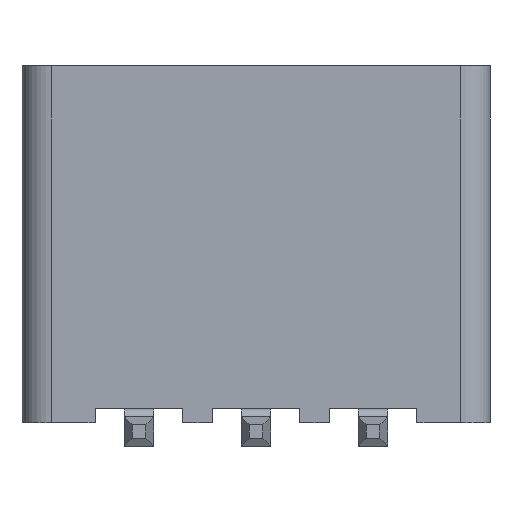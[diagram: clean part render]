
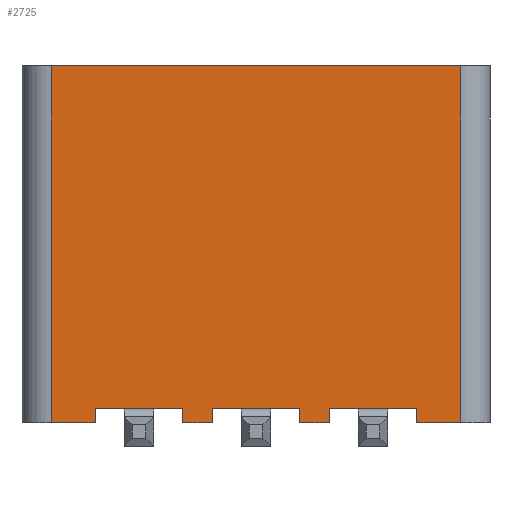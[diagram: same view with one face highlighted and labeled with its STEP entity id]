
A CAD part, front view. The second image highlights one B-rep face of the part: STEP entity #2725.
In plain terms, the highlighted planar face has unit normal (0, -1, 0).
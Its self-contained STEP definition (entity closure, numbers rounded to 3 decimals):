
#11 = ORIENTED_EDGE ( 'NONE', *, *, #2020, .T. ) ;
#19 = CARTESIAN_POINT ( 'NONE',  ( 4.75, -2.7, 0. ) ) ;
#38 = VECTOR ( 'NONE', #557, 1000. ) ;
#58 = LINE ( 'NONE', #2174, #2047 ) ;
#85 = LINE ( 'NONE', #789, #38 ) ;
#87 = LINE ( 'NONE', #790, #674 ) ;
#128 = CARTESIAN_POINT ( 'NONE',  ( 1.25, -2.7, 0.25 ) ) ;
#173 = EDGE_CURVE ( 'NONE', #2019, #825, #58, .T. ) ;
#180 = EDGE_CURVE ( 'NONE', #424, #192, #2599, .T. ) ;
#192 = VERTEX_POINT ( 'NONE', #19 ) ;
#199 = CARTESIAN_POINT ( 'NONE',  ( 5.5, -2.7, 6.1 ) ) ;
#227 = DIRECTION ( 'NONE',  ( 0., 0., -1. ) ) ;
#266 = ORIENTED_EDGE ( 'NONE', *, *, #180, .T. ) ;
#269 = EDGE_CURVE ( 'NONE', #2885, #192, #536, .T. ) ;
#272 = CARTESIAN_POINT ( 'NONE',  ( 3.25, -2.7, 0.25 ) ) ;
#284 = CARTESIAN_POINT ( 'NONE',  ( 2.75, -2.7, 0. ) ) ;
#292 = ORIENTED_EDGE ( 'NONE', *, *, #2459, .F. ) ;
#300 = EDGE_CURVE ( 'NONE', #2869, #2008, #2624, .T. ) ;
#386 = CARTESIAN_POINT ( 'NONE',  ( -0.75, -2.7, 0. ) ) ;
#424 = VERTEX_POINT ( 'NONE', #2438 ) ;
#430 = VECTOR ( 'NONE', #1028, 1000. ) ;
#444 = LINE ( 'NONE', #199, #855 ) ;
#485 = EDGE_CURVE ( 'NONE', #1780, #424, #2649, .T. ) ;
#536 = LINE ( 'NONE', #1696, #2934 ) ;
#546 = VECTOR ( 'NONE', #2665, 1000. ) ;
#548 = ORIENTED_EDGE ( 'NONE', *, *, #2623, .T. ) ;
#557 = DIRECTION ( 'NONE',  ( -1., 0., 0. ) ) ;
#564 = VECTOR ( 'NONE', #2531, 1000. ) ;
#566 = VECTOR ( 'NONE', #834, 1000. ) ;
#576 = DIRECTION ( 'NONE',  ( 0., 0., -1. ) ) ;
#588 = VERTEX_POINT ( 'NONE', #1797 ) ;
#674 = VECTOR ( 'NONE', #2382, 1000. ) ;
#732 = DIRECTION ( 'NONE',  ( 0., 0., 1. ) ) ;
#789 = CARTESIAN_POINT ( 'NONE',  ( 6., -2.7, 0. ) ) ;
#790 = CARTESIAN_POINT ( 'NONE',  ( 6., -2.7, 0. ) ) ;
#803 = LINE ( 'NONE', #2239, #2181 ) ;
#825 = VERTEX_POINT ( 'NONE', #2109 ) ;
#827 = EDGE_CURVE ( 'NONE', #2881, #2975, #3008, .T. ) ;
#834 = DIRECTION ( 'NONE',  ( 1., 0., 0. ) ) ;
#855 = VECTOR ( 'NONE', #1823, 1000. ) ;
#888 = CARTESIAN_POINT ( 'NONE',  ( 2.75, -2.7, 0.25 ) ) ;
#971 = EDGE_CURVE ( 'NONE', #2869, #2089, #85, .T. ) ;
#1028 = DIRECTION ( 'NONE',  ( 0., 0., 1. ) ) ;
#1059 = DIRECTION ( 'NONE',  ( 0., -1., 0. ) ) ;
#1067 = EDGE_CURVE ( 'NONE', #2348, #1780, #2000, .T. ) ;
#1071 = CARTESIAN_POINT ( 'NONE',  ( 2.75, -2.7, 0.25 ) ) ;
#1079 = VERTEX_POINT ( 'NONE', #1982 ) ;
#1122 = EDGE_CURVE ( 'NONE', #2106, #825, #1556, .T. ) ;
#1140 = CARTESIAN_POINT ( 'NONE',  ( -0.75, -2.7, 0.25 ) ) ;
#1199 = VECTOR ( 'NONE', #732, 1000. ) ;
#1203 = VECTOR ( 'NONE', #1545, 1000. ) ;
#1235 = CARTESIAN_POINT ( 'NONE',  ( 1.25, -2.7, 0.25 ) ) ;
#1263 = CARTESIAN_POINT ( 'NONE',  ( 3.25, -2.7, 0. ) ) ;
#1285 = CARTESIAN_POINT ( 'NONE',  ( 6., -2.7, 6.1 ) ) ;
#1304 = EDGE_CURVE ( 'NONE', #1642, #588, #2763, .T. ) ;
#1313 = DIRECTION ( 'NONE',  ( 0., 0., 1. ) ) ;
#1360 = AXIS2_PLACEMENT_3D ( 'NONE', #1285, #1059, #1375 ) ;
#1375 = DIRECTION ( 'NONE',  ( 0., 0., 1. ) ) ;
#1511 = FACE_OUTER_BOUND ( 'NONE', #2034, .T. ) ;
#1515 = EDGE_CURVE ( 'NONE', #1079, #2106, #2484, .T. ) ;
#1516 = CARTESIAN_POINT ( 'NONE',  ( 6., -2.7, 6.1 ) ) ;
#1526 = CARTESIAN_POINT ( 'NONE',  ( -0.75, -2.7, 0.25 ) ) ;
#1545 = DIRECTION ( 'NONE',  ( 0., 0., -1. ) ) ;
#1556 = LINE ( 'NONE', #2014, #1203 ) ;
#1580 = EDGE_CURVE ( 'NONE', #588, #2089, #803, .T. ) ;
#1608 = EDGE_CURVE ( 'NONE', #2885, #1079, #444, .T. ) ;
#1621 = ORIENTED_EDGE ( 'NONE', *, *, #827, .T. ) ;
#1642 = VERTEX_POINT ( 'NONE', #1140 ) ;
#1690 = CARTESIAN_POINT ( 'NONE',  ( 4.75, -2.7, 0.25 ) ) ;
#1696 = CARTESIAN_POINT ( 'NONE',  ( 6., -2.7, 0. ) ) ;
#1733 = LINE ( 'NONE', #1526, #2654 ) ;
#1752 = VECTOR ( 'NONE', #227, 1000. ) ;
#1780 = VERTEX_POINT ( 'NONE', #272 ) ;
#1797 = CARTESIAN_POINT ( 'NONE',  ( 0.75, -2.7, 0.25 ) ) ;
#1823 = DIRECTION ( 'NONE',  ( 0., 0., 1. ) ) ;
#1835 = ORIENTED_EDGE ( 'NONE', *, *, #1608, .T. ) ;
#1900 = ORIENTED_EDGE ( 'NONE', *, *, #485, .T. ) ;
#1926 = CARTESIAN_POINT ( 'NONE',  ( 2.75, -2.7, 0.25 ) ) ;
#1979 = ORIENTED_EDGE ( 'NONE', *, *, #269, .F. ) ;
#1982 = CARTESIAN_POINT ( 'NONE',  ( 5.5, -2.7, 6.1 ) ) ;
#1994 = ORIENTED_EDGE ( 'NONE', *, *, #1067, .T. ) ;
#2000 = LINE ( 'NONE', #2739, #430 ) ;
#2002 = DIRECTION ( 'NONE',  ( -1., 0., 0. ) ) ;
#2008 = VERTEX_POINT ( 'NONE', #128 ) ;
#2014 = CARTESIAN_POINT ( 'NONE',  ( -1.5, -2.7, 6.1 ) ) ;
#2019 = VERTEX_POINT ( 'NONE', #386 ) ;
#2020 = EDGE_CURVE ( 'NONE', #2008, #2881, #2938, .T. ) ;
#2023 = CARTESIAN_POINT ( 'NONE',  ( -1.5, -2.7, 6.1 ) ) ;
#2034 = EDGE_LOOP ( 'NONE', ( #266, #1979, #1835, #2757, #2552, #2651, #548, #3029, #2707, #3013, #2788, #11, #1621, #292, #1994, #1900 ) ) ;
#2047 = VECTOR ( 'NONE', #2116, 1000. ) ;
#2072 = VECTOR ( 'NONE', #2002, 1000. ) ;
#2089 = VERTEX_POINT ( 'NONE', #2263 ) ;
#2092 = CARTESIAN_POINT ( 'NONE',  ( 0.75, -2.7, 0.25 ) ) ;
#2106 = VERTEX_POINT ( 'NONE', #2023 ) ;
#2109 = CARTESIAN_POINT ( 'NONE',  ( -1.5, -2.7, 0. ) ) ;
#2116 = DIRECTION ( 'NONE',  ( -1., 0., 0. ) ) ;
#2127 = DIRECTION ( 'NONE',  ( -1., 0., 0. ) ) ;
#2174 = CARTESIAN_POINT ( 'NONE',  ( 6., -2.7, 0. ) ) ;
#2179 = CARTESIAN_POINT ( 'NONE',  ( 1.25, -2.7, 0. ) ) ;
#2181 = VECTOR ( 'NONE', #576, 1000. ) ;
#2206 = CARTESIAN_POINT ( 'NONE',  ( 4.75, -2.7, 0.25 ) ) ;
#2239 = CARTESIAN_POINT ( 'NONE',  ( 0.75, -2.7, 0.25 ) ) ;
#2263 = CARTESIAN_POINT ( 'NONE',  ( 0.75, -2.7, 0. ) ) ;
#2348 = VERTEX_POINT ( 'NONE', #1263 ) ;
#2382 = DIRECTION ( 'NONE',  ( -1., 0., 0. ) ) ;
#2412 = CARTESIAN_POINT ( 'NONE',  ( 5.5, -2.7, 0. ) ) ;
#2438 = CARTESIAN_POINT ( 'NONE',  ( 4.75, -2.7, 0.25 ) ) ;
#2459 = EDGE_CURVE ( 'NONE', #2348, #2975, #87, .T. ) ;
#2466 = PLANE ( 'NONE',  #1360 ) ;
#2484 = LINE ( 'NONE', #1516, #2072 ) ;
#2531 = DIRECTION ( 'NONE',  ( 1., 0., 0. ) ) ;
#2538 = VECTOR ( 'NONE', #2559, 1000. ) ;
#2552 = ORIENTED_EDGE ( 'NONE', *, *, #1122, .T. ) ;
#2559 = DIRECTION ( 'NONE',  ( 0., 0., -1. ) ) ;
#2599 = LINE ( 'NONE', #1690, #1752 ) ;
#2623 = EDGE_CURVE ( 'NONE', #2019, #1642, #1733, .T. ) ;
#2624 = LINE ( 'NONE', #1235, #1199 ) ;
#2649 = LINE ( 'NONE', #2206, #546 ) ;
#2651 = ORIENTED_EDGE ( 'NONE', *, *, #173, .F. ) ;
#2654 = VECTOR ( 'NONE', #1313, 1000. ) ;
#2665 = DIRECTION ( 'NONE',  ( 1., 0., 0. ) ) ;
#2707 = ORIENTED_EDGE ( 'NONE', *, *, #1580, .T. ) ;
#2725 = ADVANCED_FACE ( 'NONE', ( #1511 ), #2466, .T. ) ;
#2739 = CARTESIAN_POINT ( 'NONE',  ( 3.25, -2.7, 0.25 ) ) ;
#2757 = ORIENTED_EDGE ( 'NONE', *, *, #1515, .T. ) ;
#2763 = LINE ( 'NONE', #2092, #564 ) ;
#2788 = ORIENTED_EDGE ( 'NONE', *, *, #300, .T. ) ;
#2869 = VERTEX_POINT ( 'NONE', #2179 ) ;
#2881 = VERTEX_POINT ( 'NONE', #1926 ) ;
#2885 = VERTEX_POINT ( 'NONE', #2412 ) ;
#2934 = VECTOR ( 'NONE', #2127, 1000. ) ;
#2938 = LINE ( 'NONE', #1071, #566 ) ;
#2975 = VERTEX_POINT ( 'NONE', #284 ) ;
#3008 = LINE ( 'NONE', #888, #2538 ) ;
#3013 = ORIENTED_EDGE ( 'NONE', *, *, #971, .F. ) ;
#3029 = ORIENTED_EDGE ( 'NONE', *, *, #1304, .T. ) ;
